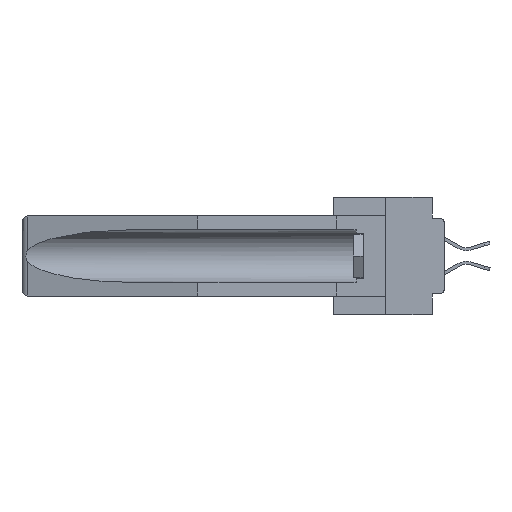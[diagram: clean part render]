
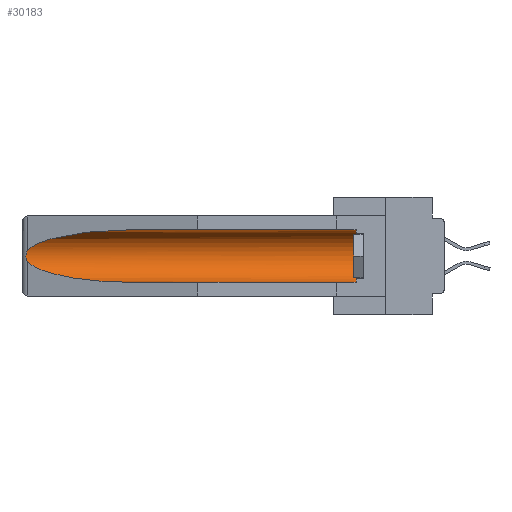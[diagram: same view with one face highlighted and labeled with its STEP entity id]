
A CAD part, left-side view. The second image highlights one B-rep face of the part: STEP entity #30183.
In plain terms, the highlighted cylindrical face has radius 2.857 mm (diameter 5.715 mm), a partial arc.
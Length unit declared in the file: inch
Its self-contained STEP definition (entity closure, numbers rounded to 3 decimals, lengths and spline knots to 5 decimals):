
#218 = CARTESIAN_POINT ( 'NONE',  ( 0.25451, 1.48313, -0.09465 ) ) ;
#918 = CARTESIAN_POINT ( 'NONE',  ( 0.155, 1.07973, -0.284 ) ) ;
#1771 = VECTOR ( 'NONE', #8511, 39.37008 ) ;
#2308 = CARTESIAN_POINT ( 'NONE',  ( 0.155, 1.07973, -0.059 ) ) ;
#2340 = CARTESIAN_POINT ( 'NONE',  ( 0.155, -0.30754, -0.059 ) ) ;
#2552 = CARTESIAN_POINT ( 'NONE',  ( 0.21114, 1.30732, -0.059 ) ) ;
#2786 = CYLINDRICAL_SURFACE ( 'NONE', #5830, 0.1125 ) ;
#2825 = CARTESIAN_POINT ( 'NONE',  ( 0.155, 1.07973, -0.284 ) ) ;
#2978 = DIRECTION ( 'NONE',  ( 0., 0., 1. ) ) ;
#3259 = VERTEX_POINT ( 'NONE', #2825 ) ;
#3335 = VERTEX_POINT ( 'NONE', #30031 ) ;
#4001 = CARTESIAN_POINT ( 'NONE',  ( 0.25451, 1.48313, -0.24835 ) ) ;
#4808 = DIRECTION ( 'NONE',  ( 0., -1., 0. ) ) ;
#5053 = CARTESIAN_POINT ( 'NONE',  ( 0.26537, 1.52718, -0.14972 ) ) ;
#5241 = CARTESIAN_POINT ( 'NONE',  ( 0.2673, 1.5327, -0.16383 ) ) ;
#5608 = CARTESIAN_POINT ( 'NONE',  ( 0.26654, 1.53092, -0.15636 ) ) ;
#5830 = AXIS2_PLACEMENT_3D ( 'NONE', #20101, #6050, #2978 ) ;
#6050 = DIRECTION ( 'NONE',  ( 0., 1., 0. ) ) ;
#6373 = CARTESIAN_POINT ( 'NONE',  ( 0.26537, 1.52718, -0.19328 ) ) ;
#8212 = FACE_OUTER_BOUND ( 'NONE', #16137, .T. ) ;
#8511 = DIRECTION ( 'NONE',  ( 0., 1., 0. ) ) ;
#9066 = ORIENTED_EDGE ( 'NONE', *, *, #16640, .T. ) ;
#9145 = VERTEX_POINT ( 'NONE', #19896 ) ;
#10162 = EDGE_CURVE ( 'NONE', #27828, #15420, #35995, .T. ) ;
#11471 = CARTESIAN_POINT ( 'NONE',  ( 0.155, -0.30754, -0.284 ) ) ;
#12763 = VERTEX_POINT ( 'NONE', #27041 ) ;
#12990 = EDGE_CURVE ( 'NONE', #3335, #27828, #37717, .T. ) ;
#14155 = AXIS2_PLACEMENT_3D ( 'NONE', #19808, #4808, #22125 ) ;
#14383 = CARTESIAN_POINT ( 'NONE',  ( 0.2675, 1.53308, -0.17534 ) ) ;
#14980 = CARTESIAN_POINT ( 'NONE',  ( 0.155, 1.07973, -0.059 ) ) ;
#15420 = VERTEX_POINT ( 'NONE', #32645 ) ;
#15492 = CARTESIAN_POINT ( 'NONE',  ( 0.21114, 1.30732, -0.284 ) ) ;
#16137 = EDGE_LOOP ( 'NONE', ( #27798, #9066, #38308, #26988, #25991, #24535 ) ) ;
#16640 = EDGE_CURVE ( 'NONE', #15420, #12763, #34395, .T. ) ;
#17117 = CARTESIAN_POINT ( 'NONE',  ( 0.2675, 1.53308, -0.16763 ) ) ;
#17486 = CARTESIAN_POINT ( 'NONE',  ( 0.2673, 1.53269, -0.17917 ) ) ;
#19808 = CARTESIAN_POINT ( 'NONE',  ( 0.155, 0.126, -0.1715 ) ) ;
#19896 = CARTESIAN_POINT ( 'NONE',  ( 0.155, 0.126, -0.284 ) ) ;
#20047 = CARTESIAN_POINT ( 'NONE',  ( 0.26597, 1.52961, -0.15275 ) ) ;
#20101 = CARTESIAN_POINT ( 'NONE',  ( 0.155, -0.30754, -0.1715 ) ) ;
#20926 = CARTESIAN_POINT ( 'NONE',  ( 0.26537, 1.52718, -0.19328 ) ) ;
#21367 = CARTESIAN_POINT ( 'NONE',  ( 0.26597, 1.5296, -0.19026 ) ) ;
#22125 = DIRECTION ( 'NONE',  ( 0., 0., 1. ) ) ;
#23056 = VECTOR ( 'NONE', #23353, 39.37008 ) ;
#23353 = DIRECTION ( 'NONE',  ( 0., 1., 0. ) ) ;
#24535 = ORIENTED_EDGE ( 'NONE', *, *, #12990, .T. ) ;
#25258 = EDGE_CURVE ( 'NONE', #9145, #3259, #27232, .T. ) ;
#25991 = ORIENTED_EDGE ( 'NONE', *, *, #35350, .T. ) ;
#26836 = CARTESIAN_POINT ( 'NONE',  ( 0.26537, 1.52718, -0.14972 ) ) ;
#26988 = ORIENTED_EDGE ( 'NONE', *, *, #25258, .F. ) ;
#27041 = CARTESIAN_POINT ( 'NONE',  ( 0.26537, 1.52718, -0.19328 ) ) ;
#27232 = LINE ( 'NONE', #11471, #23056 ) ;
#27798 = ORIENTED_EDGE ( 'NONE', *, *, #10162, .T. ) ;
#27828 = VERTEX_POINT ( 'NONE', #2308 ) ;
#30031 = CARTESIAN_POINT ( 'NONE',  ( 0.155, 0.126, -0.059 ) ) ;
#30183 = ADVANCED_FACE ( 'NONE', ( #8212 ), #2786, .F. ) ;
#30919 = CIRCLE ( 'NONE', #14155, 0.1125 ) ;
#32645 = CARTESIAN_POINT ( 'NONE',  ( 0.26537, 1.52718, -0.14972 ) ) ;
#33252 =( BOUNDED_CURVE ( )  B_SPLINE_CURVE ( 3, ( #20926, #4001, #15492, #918 ),
 .UNSPECIFIED., .F., .F. ) 
 B_SPLINE_CURVE_WITH_KNOTS ( ( 4, 4 ),
 ( 0.1948, 1.5708 ),
 .UNSPECIFIED. ) 
 CURVE ( )  GEOMETRIC_REPRESENTATION_ITEM ( )  RATIONAL_B_SPLINE_CURVE ( ( 1., 0.848, 0.848, 1. ) ) 
 REPRESENTATION_ITEM ( '' )  );
#34395 = B_SPLINE_CURVE_WITH_KNOTS ( 'NONE', 3,
 ( #5053, #20047, #5608, #5241, #17117, #14383, #17486, #38120, #21367, #6373 ),
 .UNSPECIFIED., .F., .F.,
 ( 4, 2, 2, 2, 4 ),
 ( 0., 0.00029, 0.00058, 0.00087, 0.00117 ),
 .UNSPECIFIED. ) ;
#35350 = EDGE_CURVE ( 'NONE', #9145, #3335, #30919, .T. ) ;
#35517 = EDGE_CURVE ( 'NONE', #12763, #3259, #33252, .T. ) ;
#35995 =( BOUNDED_CURVE ( )  B_SPLINE_CURVE ( 3, ( #14980, #2552, #218, #26836 ),
 .UNSPECIFIED., .F., .F. ) 
 B_SPLINE_CURVE_WITH_KNOTS ( ( 4, 4 ),
 ( 4.71239, 6.08839 ),
 .UNSPECIFIED. ) 
 CURVE ( )  GEOMETRIC_REPRESENTATION_ITEM ( )  RATIONAL_B_SPLINE_CURVE ( ( 1., 0.848, 0.848, 1. ) ) 
 REPRESENTATION_ITEM ( '' )  );
#37717 = LINE ( 'NONE', #2340, #1771 ) ;
#38120 = CARTESIAN_POINT ( 'NONE',  ( 0.26655, 1.53094, -0.18657 ) ) ;
#38308 = ORIENTED_EDGE ( 'NONE', *, *, #35517, .T. ) ;
